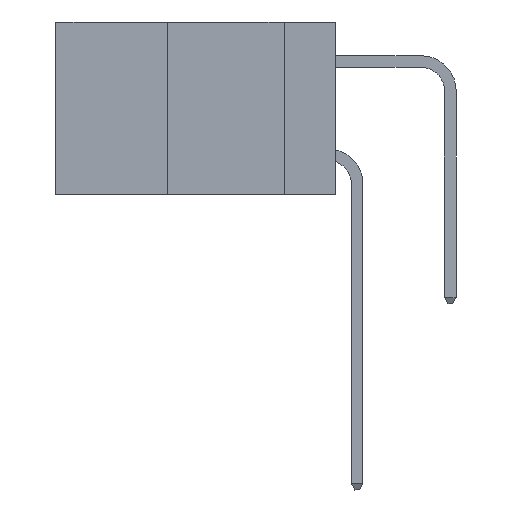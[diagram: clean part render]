
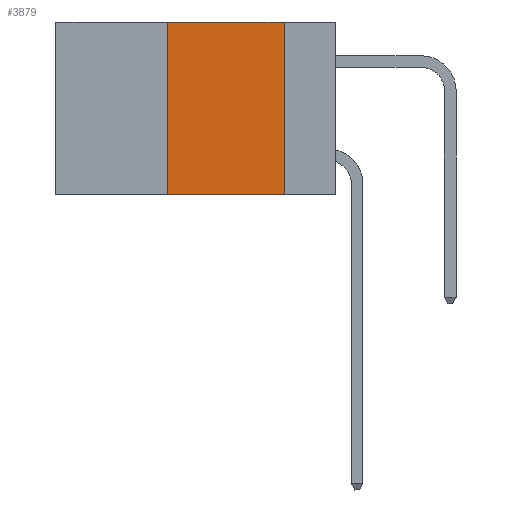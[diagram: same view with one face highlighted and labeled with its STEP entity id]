
A CAD part, left-side view. The second image highlights one B-rep face of the part: STEP entity #3879.
In plain terms, the highlighted planar face has unit normal (-1, 0, 0).
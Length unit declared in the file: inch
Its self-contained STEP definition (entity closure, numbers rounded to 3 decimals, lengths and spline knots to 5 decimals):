
#659 = LINE ( 'NONE', #14549, #1426 ) ;
#1426 = VECTOR ( 'NONE', #21258, 39.37008 ) ;
#2178 = CARTESIAN_POINT ( 'NONE',  ( 0., 0.36, -0.37 ) ) ;
#3047 = VECTOR ( 'NONE', #12975, 39.37008 ) ;
#3879 = ADVANCED_FACE ( 'NONE', ( #17738 ), #11591, .F. ) ;
#4259 = DIRECTION ( 'NONE',  ( 0., -1., 0. ) ) ;
#4687 = DIRECTION ( 'NONE',  ( 1., 0., 0. ) ) ;
#4873 = CARTESIAN_POINT ( 'NONE',  ( 0., 0.6, 0. ) ) ;
#5529 = ORIENTED_EDGE ( 'NONE', *, *, #15431, .F. ) ;
#6408 = DIRECTION ( 'NONE',  ( 0., 0., -1. ) ) ;
#8021 = EDGE_CURVE ( 'NONE', #9495, #22520, #22549, .T. ) ;
#9222 = LINE ( 'NONE', #26654, #3047 ) ;
#9442 = DIRECTION ( 'NONE',  ( 0., 0., -1. ) ) ;
#9495 = VERTEX_POINT ( 'NONE', #14330 ) ;
#9603 = ORIENTED_EDGE ( 'NONE', *, *, #25614, .F. ) ;
#11591 = PLANE ( 'NONE',  #28648 ) ;
#12579 = EDGE_CURVE ( 'NONE', #21091, #22520, #9222, .T. ) ;
#12975 = DIRECTION ( 'NONE',  ( 0., -1., 0. ) ) ;
#14027 = ORIENTED_EDGE ( 'NONE', *, *, #12579, .T. ) ;
#14330 = CARTESIAN_POINT ( 'NONE',  ( 0., 0.11, 0. ) ) ;
#14549 = CARTESIAN_POINT ( 'NONE',  ( 0., 0.36, 0. ) ) ;
#14751 = CARTESIAN_POINT ( 'NONE',  ( 0., 0.36, 0. ) ) ;
#14941 = CARTESIAN_POINT ( 'NONE',  ( 0., 0.11, 0. ) ) ;
#15431 = EDGE_CURVE ( 'NONE', #21091, #25466, #659, .T. ) ;
#16217 = CARTESIAN_POINT ( 'NONE',  ( 0., 0.11, -0.37 ) ) ;
#17738 = FACE_OUTER_BOUND ( 'NONE', #26790, .T. ) ;
#18549 = LINE ( 'NONE', #29722, #28686 ) ;
#21091 = VERTEX_POINT ( 'NONE', #2178 ) ;
#21258 = DIRECTION ( 'NONE',  ( 0., 0., 1. ) ) ;
#21525 = ORIENTED_EDGE ( 'NONE', *, *, #8021, .F. ) ;
#22520 = VERTEX_POINT ( 'NONE', #16217 ) ;
#22549 = LINE ( 'NONE', #14941, #24724 ) ;
#24724 = VECTOR ( 'NONE', #6408, 39.37008 ) ;
#25466 = VERTEX_POINT ( 'NONE', #14751 ) ;
#25614 = EDGE_CURVE ( 'NONE', #25466, #9495, #18549, .T. ) ;
#26654 = CARTESIAN_POINT ( 'NONE',  ( 0., 0.6, -0.37 ) ) ;
#26790 = EDGE_LOOP ( 'NONE', ( #21525, #9603, #5529, #14027 ) ) ;
#28648 = AXIS2_PLACEMENT_3D ( 'NONE', #4873, #4687, #9442 ) ;
#28686 = VECTOR ( 'NONE', #4259, 39.37008 ) ;
#29722 = CARTESIAN_POINT ( 'NONE',  ( 0., 0.6, 0. ) ) ;
